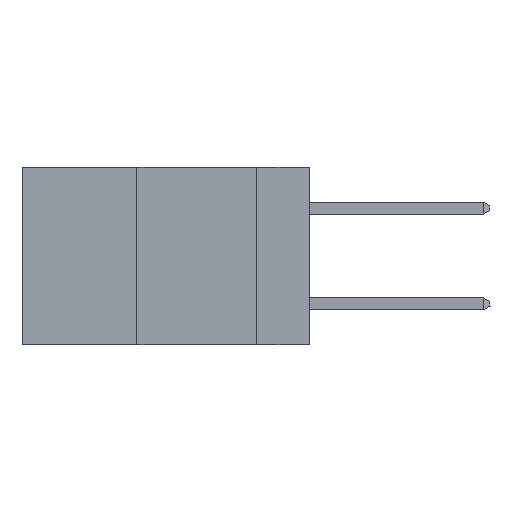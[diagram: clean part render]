
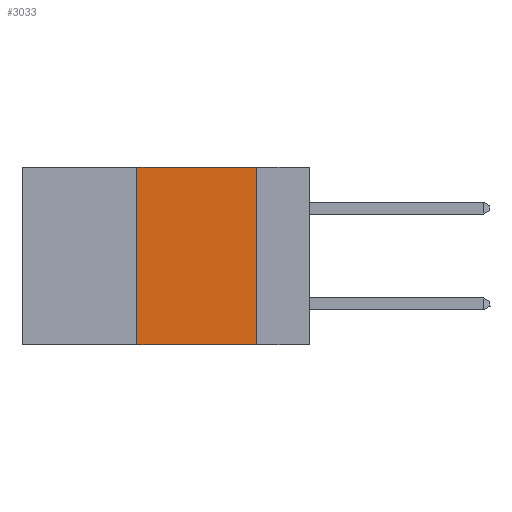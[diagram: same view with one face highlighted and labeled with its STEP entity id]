
A CAD part, left-side view. The second image highlights one B-rep face of the part: STEP entity #3033.
In plain terms, the highlighted planar face has unit normal (-1, 0, 0).
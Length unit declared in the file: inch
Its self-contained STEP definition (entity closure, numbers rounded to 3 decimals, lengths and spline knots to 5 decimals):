
#1043 = VECTOR ( 'NONE', #17764, 39.37008 ) ;
#1098 = LINE ( 'NONE', #21760, #12085 ) ;
#1656 = CARTESIAN_POINT ( 'NONE',  ( 0., 0.6, -0.37 ) ) ;
#1707 = EDGE_CURVE ( 'NONE', #6698, #25783, #1098, .T. ) ;
#3033 = ADVANCED_FACE ( 'NONE', ( #17387 ), #17949, .F. ) ;
#3139 = ORIENTED_EDGE ( 'NONE', *, *, #10285, .F. ) ;
#5535 = CARTESIAN_POINT ( 'NONE',  ( 0., 0.11, -0.37 ) ) ;
#5655 = DIRECTION ( 'NONE',  ( 0., -1., 0. ) ) ;
#6698 = VERTEX_POINT ( 'NONE', #20669 ) ;
#7852 = CARTESIAN_POINT ( 'NONE',  ( 0., 0.11, 0. ) ) ;
#8083 = CARTESIAN_POINT ( 'NONE',  ( 0., 0.6, 0. ) ) ;
#8367 = VERTEX_POINT ( 'NONE', #5535 ) ;
#9091 = EDGE_LOOP ( 'NONE', ( #14369, #16766, #3139, #9444 ) ) ;
#9444 = ORIENTED_EDGE ( 'NONE', *, *, #24050, .T. ) ;
#10285 = EDGE_CURVE ( 'NONE', #12655, #6698, #20653, .T. ) ;
#10931 = CARTESIAN_POINT ( 'NONE',  ( 0., 0.11, 0. ) ) ;
#11056 = DIRECTION ( 'NONE',  ( 0., 0., 1. ) ) ;
#12085 = VECTOR ( 'NONE', #5655, 39.37008 ) ;
#12153 = CARTESIAN_POINT ( 'NONE',  ( 0., 0.36, -0.37 ) ) ;
#12655 = VERTEX_POINT ( 'NONE', #12153 ) ;
#13661 = DIRECTION ( 'NONE',  ( 0., 0., -1. ) ) ;
#14369 = ORIENTED_EDGE ( 'NONE', *, *, #16315, .F. ) ;
#16173 = DIRECTION ( 'NONE',  ( 1., 0., 0. ) ) ;
#16315 = EDGE_CURVE ( 'NONE', #25783, #8367, #22280, .T. ) ;
#16766 = ORIENTED_EDGE ( 'NONE', *, *, #1707, .F. ) ;
#16959 = VECTOR ( 'NONE', #13661, 39.37008 ) ;
#17387 = FACE_OUTER_BOUND ( 'NONE', #9091, .T. ) ;
#17407 = LINE ( 'NONE', #1656, #1043 ) ;
#17764 = DIRECTION ( 'NONE',  ( 0., -1., 0. ) ) ;
#17949 = PLANE ( 'NONE',  #18839 ) ;
#18839 = AXIS2_PLACEMENT_3D ( 'NONE', #8083, #16173, #24400 ) ;
#18963 = CARTESIAN_POINT ( 'NONE',  ( 0., 0.36, 0. ) ) ;
#20653 = LINE ( 'NONE', #18963, #24415 ) ;
#20669 = CARTESIAN_POINT ( 'NONE',  ( 0., 0.36, 0. ) ) ;
#21760 = CARTESIAN_POINT ( 'NONE',  ( 0., 0.6, 0. ) ) ;
#22280 = LINE ( 'NONE', #7852, #16959 ) ;
#24050 = EDGE_CURVE ( 'NONE', #12655, #8367, #17407, .T. ) ;
#24400 = DIRECTION ( 'NONE',  ( 0., 0., -1. ) ) ;
#24415 = VECTOR ( 'NONE', #11056, 39.37008 ) ;
#25783 = VERTEX_POINT ( 'NONE', #10931 ) ;
